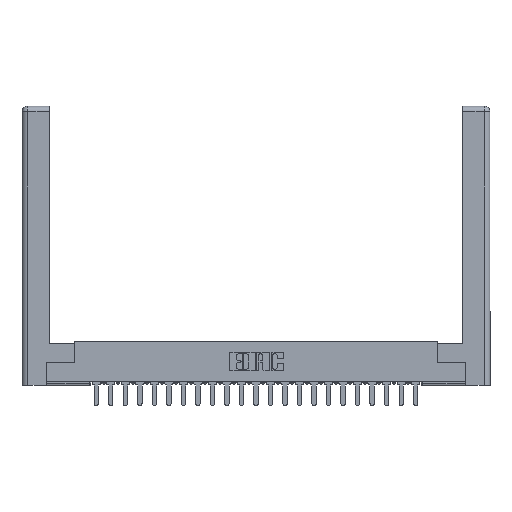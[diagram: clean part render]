
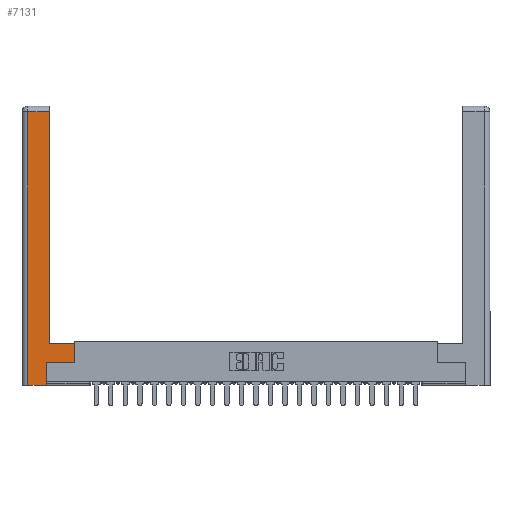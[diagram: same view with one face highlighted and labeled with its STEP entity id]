
A CAD part, top view. The second image highlights one B-rep face of the part: STEP entity #7131.
In plain terms, the highlighted planar face has unit normal (0, 0, 1).
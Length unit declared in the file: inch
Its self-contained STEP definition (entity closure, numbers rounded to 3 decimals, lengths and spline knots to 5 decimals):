
#168 = ORIENTED_EDGE ( 'NONE', *, *, #14338, .T. ) ;
#740 = LINE ( 'NONE', #24266, #19821 ) ;
#2008 = DIRECTION ( 'NONE',  ( 0., 0., -1. ) ) ;
#2608 = CARTESIAN_POINT ( 'NONE',  ( 0.265, 0.245, 0. ) ) ;
#2803 = VECTOR ( 'NONE', #18600, 39.37008 ) ;
#2976 = EDGE_CURVE ( 'NONE', #12622, #16877, #7879, .T. ) ;
#3126 = LINE ( 'NONE', #2608, #15901 ) ;
#3187 = CARTESIAN_POINT ( 'NONE',  ( 0.0615, 2.94, 0. ) ) ;
#3595 = DIRECTION ( 'NONE',  ( 1., 0., 0. ) ) ;
#3629 = CARTESIAN_POINT ( 'NONE',  ( 0., 0., 0. ) ) ;
#3940 = VERTEX_POINT ( 'NONE', #12210 ) ;
#4091 = LINE ( 'NONE', #5411, #10330 ) ;
#4898 = VECTOR ( 'NONE', #17670, 39.37008 ) ;
#5302 = CARTESIAN_POINT ( 'NONE',  ( 0.295, 2.94, 0. ) ) ;
#5411 = CARTESIAN_POINT ( 'NONE',  ( 0.265, 0., 0. ) ) ;
#5782 = CARTESIAN_POINT ( 'NONE',  ( 0.565, 0.45, 0. ) ) ;
#5980 = ORIENTED_EDGE ( 'NONE', *, *, #19428, .T. ) ;
#6495 = VERTEX_POINT ( 'NONE', #24153 ) ;
#7131 = ADVANCED_FACE ( 'NONE', ( #9507 ), #11281, .F. ) ;
#7246 = CARTESIAN_POINT ( 'NONE',  ( 0.565, 0.245, 0. ) ) ;
#7879 = LINE ( 'NONE', #3187, #2803 ) ;
#7971 = CARTESIAN_POINT ( 'NONE',  ( 0.565, 0.45, 0. ) ) ;
#8081 = EDGE_CURVE ( 'NONE', #6495, #18125, #4091, .T. ) ;
#8206 = VECTOR ( 'NONE', #12434, 39.37008 ) ;
#8428 = DIRECTION ( 'NONE',  ( 0., 1., 0. ) ) ;
#9087 = ORIENTED_EDGE ( 'NONE', *, *, #10044, .T. ) ;
#9166 = EDGE_CURVE ( 'NONE', #23208, #22608, #14099, .T. ) ;
#9507 = FACE_OUTER_BOUND ( 'NONE', #20245, .T. ) ;
#9701 = CARTESIAN_POINT ( 'NONE',  ( 0.0615, 0., 0. ) ) ;
#9716 = EDGE_CURVE ( 'NONE', #22608, #16258, #23929, .T. ) ;
#10044 = EDGE_CURVE ( 'NONE', #18125, #23208, #3126, .T. ) ;
#10330 = VECTOR ( 'NONE', #22544, 39.37008 ) ;
#11281 = PLANE ( 'NONE',  #23027 ) ;
#11337 = CARTESIAN_POINT ( 'NONE',  ( 0.0615, 2.94, 0. ) ) ;
#11771 = VECTOR ( 'NONE', #23009, 39.37008 ) ;
#12060 = CARTESIAN_POINT ( 'NONE',  ( 0.265, 0., 0. ) ) ;
#12210 = CARTESIAN_POINT ( 'NONE',  ( 0.295, 0.45, 0. ) ) ;
#12434 = DIRECTION ( 'NONE',  ( 0., 1., 0. ) ) ;
#12622 = VERTEX_POINT ( 'NONE', #5302 ) ;
#12625 = ORIENTED_EDGE ( 'NONE', *, *, #2976, .T. ) ;
#12630 = ORIENTED_EDGE ( 'NONE', *, *, #19702, .T. ) ;
#12984 = LINE ( 'NONE', #9701, #11771 ) ;
#14099 = LINE ( 'NONE', #7246, #20981 ) ;
#14338 = EDGE_CURVE ( 'NONE', #16258, #3940, #740, .T. ) ;
#14527 = ORIENTED_EDGE ( 'NONE', *, *, #9166, .T. ) ;
#15901 = VECTOR ( 'NONE', #8428, 39.37008 ) ;
#15963 = ORIENTED_EDGE ( 'NONE', *, *, #8081, .T. ) ;
#16258 = VERTEX_POINT ( 'NONE', #5782 ) ;
#16867 = DIRECTION ( 'NONE',  ( -1., 0., 0. ) ) ;
#16877 = VERTEX_POINT ( 'NONE', #11337 ) ;
#17670 = DIRECTION ( 'NONE',  ( 0., 1., 0. ) ) ;
#18118 = CARTESIAN_POINT ( 'NONE',  ( 0.295, 3., 0. ) ) ;
#18125 = VERTEX_POINT ( 'NONE', #12060 ) ;
#18600 = DIRECTION ( 'NONE',  ( -1., 0., 0. ) ) ;
#19428 = EDGE_CURVE ( 'NONE', #3940, #12622, #23997, .T. ) ;
#19702 = EDGE_CURVE ( 'NONE', #16877, #6495, #12984, .T. ) ;
#19821 = VECTOR ( 'NONE', #20263, 39.37008 ) ;
#20245 = EDGE_LOOP ( 'NONE', ( #5980, #12625, #12630, #15963, #9087, #14527, #21735, #168 ) ) ;
#20263 = DIRECTION ( 'NONE',  ( -1., 0., 0. ) ) ;
#20981 = VECTOR ( 'NONE', #3595, 39.37008 ) ;
#21643 = CARTESIAN_POINT ( 'NONE',  ( 0.265, 0.245, 0. ) ) ;
#21735 = ORIENTED_EDGE ( 'NONE', *, *, #9716, .T. ) ;
#22544 = DIRECTION ( 'NONE',  ( 1., 0., 0. ) ) ;
#22608 = VERTEX_POINT ( 'NONE', #23755 ) ;
#23009 = DIRECTION ( 'NONE',  ( 0., -1., 0. ) ) ;
#23027 = AXIS2_PLACEMENT_3D ( 'NONE', #3629, #2008, #16867 ) ;
#23208 = VERTEX_POINT ( 'NONE', #21643 ) ;
#23755 = CARTESIAN_POINT ( 'NONE',  ( 0.565, 0.245, 0. ) ) ;
#23929 = LINE ( 'NONE', #7971, #4898 ) ;
#23997 = LINE ( 'NONE', #18118, #8206 ) ;
#24153 = CARTESIAN_POINT ( 'NONE',  ( 0.0615, 0., 0. ) ) ;
#24266 = CARTESIAN_POINT ( 'NONE',  ( 0.295, 0.45, 0. ) ) ;
